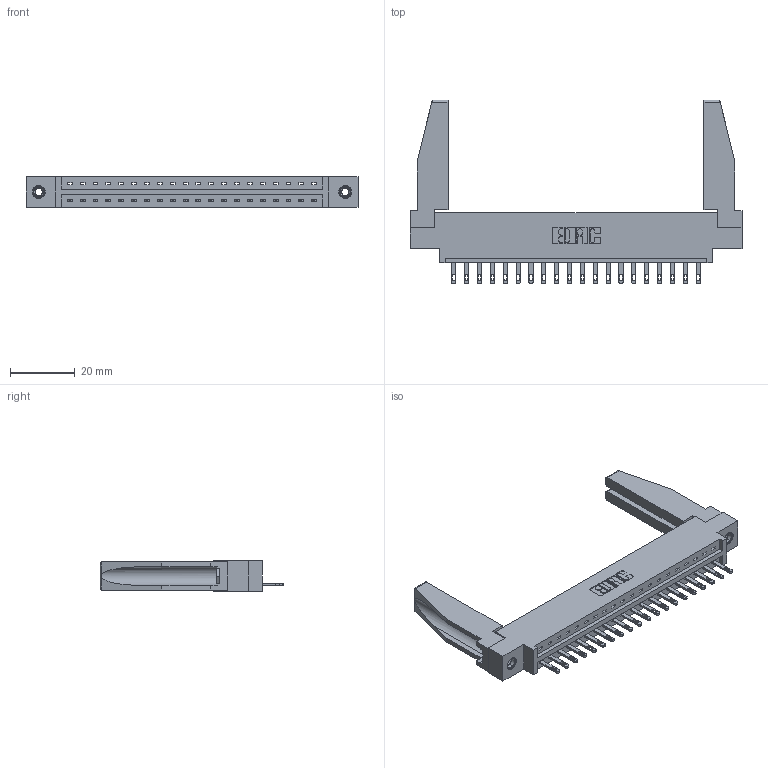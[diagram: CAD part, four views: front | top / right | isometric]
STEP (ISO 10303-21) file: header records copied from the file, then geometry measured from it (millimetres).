
FILE_DESCRIPTION (( 'STEP AP203' ), '1' );
FILE_NAME ('337-020-500-678.STEP', '2019-09-28T22:19:55', ( '' ), ( '' ), 'SwSTEP 2.0', 'SolidWorks 2016', '' );
FILE_SCHEMA (( 'CONFIG_CONTROL_DESIGN' ));
Length unit declared in the file: inch
Products named in the file (5): 337-020-500-678; 345-292-001_345-293-100; 345-250-001_345-250-001-102; 307-220-078; 337 Part_0.170 Offset - 0.156 Dia-TI
Assembly tree (25 placements, depth 2):
  337-020-500-678
    337 Part_0.170 Offset - 0.156 Dia-TI
    345-292-001_345-293-100  x20
    345-250-001_345-250-001-102  x2
    307-220-078  x2
Bounding box: 102.26 x 56.65 x 9.4 mm (x, y, z)
Volume: 14241.1 mm3; surface area: 14447.5 mm2
Topology: 25 solids, 25 shells, 1408 faces, 4253 edges, 2826 vertices
Faces by surface type: plane 958, cylinder 434, cone 12, torus 4
Entity records: 20214 total; most frequent: CARTESIAN_POINT 3512, ORIENTED_EDGE 3424, DIRECTION 3012, EDGE_CURVE 1712, LINE 1542, VECTOR 1542, VERTEX_POINT 1136, AXIS2_PLACEMENT_3D 735
